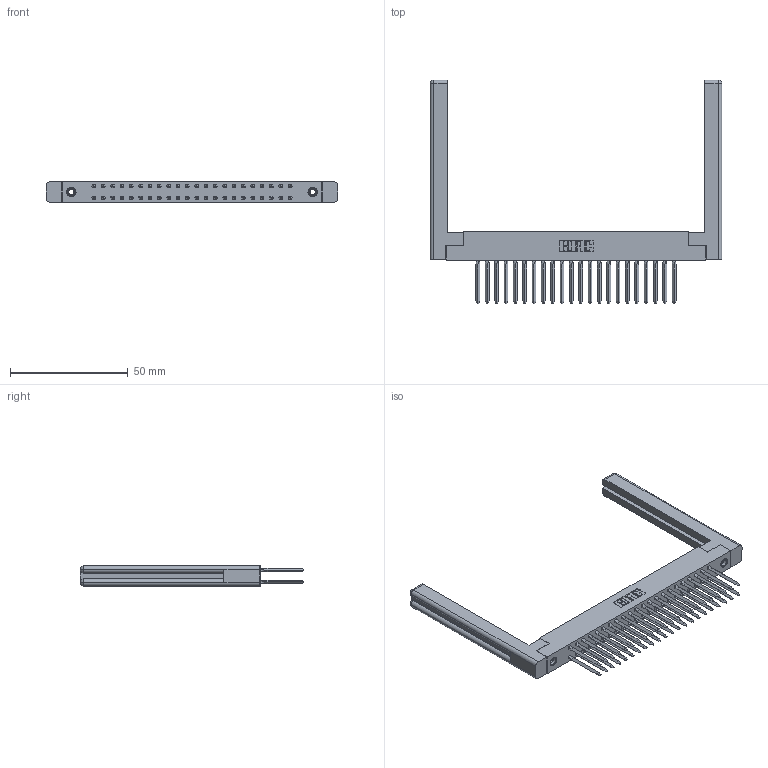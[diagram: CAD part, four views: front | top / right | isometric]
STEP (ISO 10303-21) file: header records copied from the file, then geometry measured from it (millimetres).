
FILE_DESCRIPTION (( 'STEP AP203' ), '1' );
FILE_NAME ('338-044-541-278.STEP', '2020-03-24T18:44:39', ( '' ), ( '' ), 'SwSTEP 2.0', 'SolidWorks 2016', '' );
FILE_SCHEMA (( 'CONFIG_CONTROL_DESIGN' ));
Length unit declared in the file: inch
Products named in the file (5): 338-210-001_338-210-022-004; 338-290-001_541; 345-250-001_345-250-001-102; 338-044-541-278; 307-220-058
Assembly tree (49 placements, depth 2):
  338-044-541-278
    338-210-001_338-210-022-004
    338-290-001_541  x44
    345-250-001_345-250-001-102  x2
    307-220-058  x2
Bounding box: 123.8 x 94.87 x 8.71 mm (x, y, z)
Volume: 17040.4 mm3; surface area: 22316.5 mm2
Topology: 49 solids, 49 shells, 3184 faces, 8525 edges, 5406 vertices
Faces by surface type: plane 2202, cylinder 782, bspline 176, cone 12, torus 12
Entity records: 47613 total; most frequent: CARTESIAN_POINT 9395, ORIENTED_EDGE 7874, DIRECTION 7416, EDGE_CURVE 3937, VECTOR 2926, LINE 2926, VERTEX_POINT 2554, AXIS2_PLACEMENT_3D 2245
